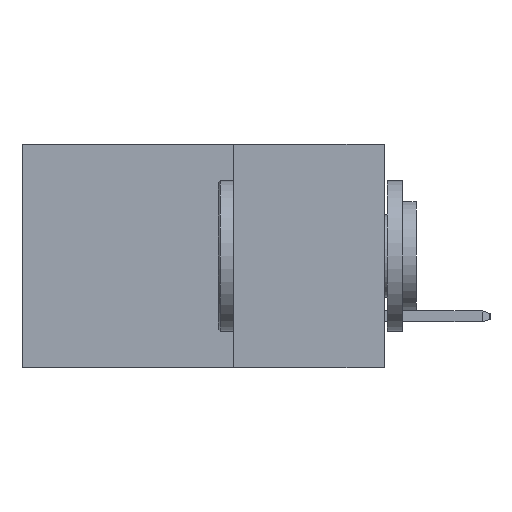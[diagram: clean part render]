
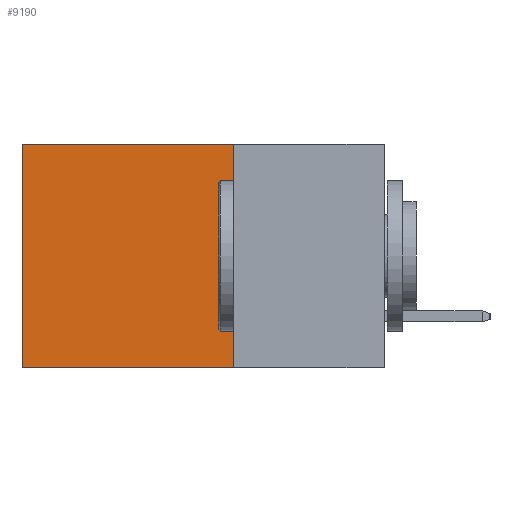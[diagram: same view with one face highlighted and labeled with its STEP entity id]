
A CAD part, left-side view. The second image highlights one B-rep face of the part: STEP entity #9190.
In plain terms, the highlighted planar face has unit normal (-1, 0, 0).
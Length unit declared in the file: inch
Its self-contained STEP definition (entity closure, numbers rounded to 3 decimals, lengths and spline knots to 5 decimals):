
#187 = VECTOR ( 'NONE', #9628, 39.37008 ) ;
#234 = FACE_OUTER_BOUND ( 'NONE', #6476, .T. ) ;
#319 = VERTEX_POINT ( 'NONE', #4714 ) ;
#604 = VECTOR ( 'NONE', #12528, 39.37008 ) ;
#961 = DIRECTION ( 'NONE',  ( 0., 0., -1. ) ) ;
#1530 = LINE ( 'NONE', #11903, #1874 ) ;
#1874 = VECTOR ( 'NONE', #2050, 39.37008 ) ;
#2050 = DIRECTION ( 'NONE',  ( 0., 1., 0. ) ) ;
#2516 = ORIENTED_EDGE ( 'NONE', *, *, #12164, .T. ) ;
#3878 = EDGE_CURVE ( 'NONE', #7567, #7975, #10705, .T. ) ;
#4004 = CARTESIAN_POINT ( 'NONE',  ( 0.298, 0.25, 0. ) ) ;
#4229 = ORIENTED_EDGE ( 'NONE', *, *, #5116, .F. ) ;
#4714 = CARTESIAN_POINT ( 'NONE',  ( 0.298, 0.25, -0.37 ) ) ;
#5116 = EDGE_CURVE ( 'NONE', #319, #7975, #1530, .T. ) ;
#5495 = VECTOR ( 'NONE', #9801, 39.37008 ) ;
#6354 = ORIENTED_EDGE ( 'NONE', *, *, #12681, .F. ) ;
#6476 = EDGE_LOOP ( 'NONE', ( #8892, #4229, #6354, #2516 ) ) ;
#6763 = AXIS2_PLACEMENT_3D ( 'NONE', #12831, #7291, #961 ) ;
#6880 = CARTESIAN_POINT ( 'NONE',  ( 0.298, 0.25, 0. ) ) ;
#6915 = CARTESIAN_POINT ( 'NONE',  ( 0.298, 0.25, 0. ) ) ;
#7291 = DIRECTION ( 'NONE',  ( 1., 0., 0. ) ) ;
#7567 = VERTEX_POINT ( 'NONE', #12698 ) ;
#7743 = CARTESIAN_POINT ( 'NONE',  ( 0.298, 0.6, -0.37 ) ) ;
#7975 = VERTEX_POINT ( 'NONE', #7743 ) ;
#8493 = LINE ( 'NONE', #6880, #5495 ) ;
#8892 = ORIENTED_EDGE ( 'NONE', *, *, #3878, .T. ) ;
#9190 = ADVANCED_FACE ( 'NONE', ( #234 ), #11029, .F. ) ;
#9603 = CARTESIAN_POINT ( 'NONE',  ( 0.298, 0.6, 0. ) ) ;
#9628 = DIRECTION ( 'NONE',  ( 0., 0., -1. ) ) ;
#9801 = DIRECTION ( 'NONE',  ( 0., 1., 0. ) ) ;
#10705 = LINE ( 'NONE', #9603, #187 ) ;
#11029 = PLANE ( 'NONE',  #6763 ) ;
#11343 = LINE ( 'NONE', #6915, #604 ) ;
#11399 = VERTEX_POINT ( 'NONE', #4004 ) ;
#11903 = CARTESIAN_POINT ( 'NONE',  ( 0.298, 0.25, -0.37 ) ) ;
#12164 = EDGE_CURVE ( 'NONE', #11399, #7567, #8493, .T. ) ;
#12528 = DIRECTION ( 'NONE',  ( 0., 0., -1. ) ) ;
#12681 = EDGE_CURVE ( 'NONE', #11399, #319, #11343, .T. ) ;
#12698 = CARTESIAN_POINT ( 'NONE',  ( 0.298, 0.6, 0. ) ) ;
#12831 = CARTESIAN_POINT ( 'NONE',  ( 0.298, 0.25, 0. ) ) ;
